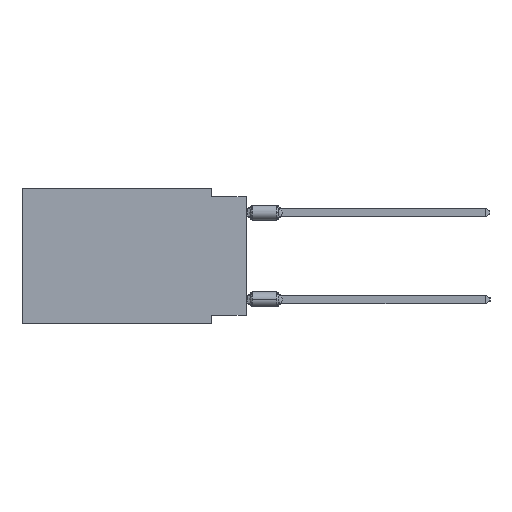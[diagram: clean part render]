
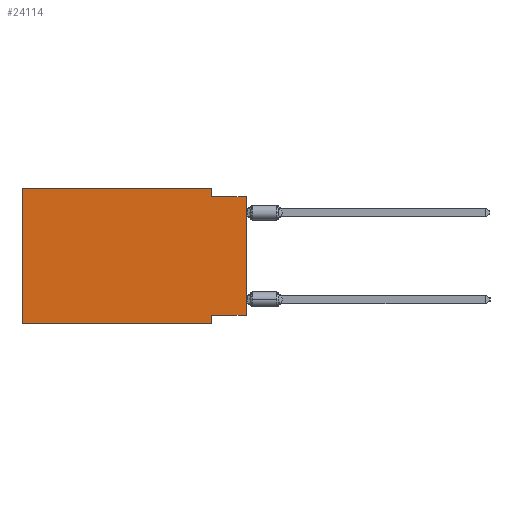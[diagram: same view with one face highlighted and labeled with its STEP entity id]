
A CAD part, left-side view. The second image highlights one B-rep face of the part: STEP entity #24114.
In plain terms, the highlighted planar face has unit normal (-1, 0, 0).
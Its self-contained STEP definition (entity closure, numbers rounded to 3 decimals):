
#54 = ORIENTED_EDGE ( 'NONE', *, *, #23808, .F. ) ;
#677 = VECTOR ( 'NONE', #4953, 1000. ) ;
#1441 = VERTEX_POINT ( 'NONE', #38375 ) ;
#1589 = LINE ( 'NONE', #32729, #54582 ) ;
#2730 = VERTEX_POINT ( 'NONE', #16091 ) ;
#4953 = DIRECTION ( 'NONE',  ( 0., 0., -1. ) ) ;
#5480 = DIRECTION ( 'NONE',  ( 0., -1., 0. ) ) ;
#6101 = ORIENTED_EDGE ( 'NONE', *, *, #49545, .F. ) ;
#6258 = EDGE_LOOP ( 'NONE', ( #31792, #54, #37159, #52309, #41253, #50559, #6101, #54483 ) ) ;
#8408 = CARTESIAN_POINT ( 'NONE',  ( 0., 0., -0.635 ) ) ;
#11209 = LINE ( 'NONE', #42965, #44977 ) ;
#12343 = VECTOR ( 'NONE', #34925, 1000. ) ;
#15864 = DIRECTION ( 'NONE',  ( 1., 0., 0. ) ) ;
#15942 = VECTOR ( 'NONE', #33941, 1000. ) ;
#16091 = CARTESIAN_POINT ( 'NONE',  ( 0., 2.54, 0. ) ) ;
#16144 = FACE_OUTER_BOUND ( 'NONE', #6258, .T. ) ;
#16253 = CARTESIAN_POINT ( 'NONE',  ( 0., 0., -0.635 ) ) ;
#19783 = CARTESIAN_POINT ( 'NONE',  ( 0., 0., -9.271 ) ) ;
#20161 = CARTESIAN_POINT ( 'NONE',  ( 0., 0., -9.271 ) ) ;
#20338 = LINE ( 'NONE', #52939, #46382 ) ;
#22613 = VECTOR ( 'NONE', #27285, 1000. ) ;
#23752 = VERTEX_POINT ( 'NONE', #25787 ) ;
#23808 = EDGE_CURVE ( 'NONE', #23752, #26547, #26990, .T. ) ;
#24114 = ADVANCED_FACE ( 'NONE', ( #16144 ), #25144, .F. ) ;
#24115 = CARTESIAN_POINT ( 'NONE',  ( 0., 16.383, -9.906 ) ) ;
#25144 = PLANE ( 'NONE',  #25330 ) ;
#25330 = AXIS2_PLACEMENT_3D ( 'NONE', #47614, #15864, #38909 ) ;
#25787 = CARTESIAN_POINT ( 'NONE',  ( 0., 2.54, -0.635 ) ) ;
#26547 = VERTEX_POINT ( 'NONE', #16253 ) ;
#26990 = LINE ( 'NONE', #8408, #22613 ) ;
#27131 = LINE ( 'NONE', #54372, #677 ) ;
#27285 = DIRECTION ( 'NONE',  ( 0., -1., 0. ) ) ;
#29143 = EDGE_CURVE ( 'NONE', #39453, #26547, #58256, .T. ) ;
#29194 = EDGE_CURVE ( 'NONE', #2730, #23752, #39709, .T. ) ;
#29446 = VERTEX_POINT ( 'NONE', #24115 ) ;
#31662 = VERTEX_POINT ( 'NONE', #49629 ) ;
#31792 = ORIENTED_EDGE ( 'NONE', *, *, #29143, .T. ) ;
#32729 = CARTESIAN_POINT ( 'NONE',  ( 0., 16.383, -9.906 ) ) ;
#33104 = DIRECTION ( 'NONE',  ( 0., -1., 0. ) ) ;
#33941 = DIRECTION ( 'NONE',  ( 0., 1., 0. ) ) ;
#34925 = DIRECTION ( 'NONE',  ( 0., 0., 1. ) ) ;
#36777 = EDGE_CURVE ( 'NONE', #31662, #2730, #11209, .T. ) ;
#37159 = ORIENTED_EDGE ( 'NONE', *, *, #29194, .F. ) ;
#37200 = VECTOR ( 'NONE', #57974, 1000. ) ;
#37273 = EDGE_CURVE ( 'NONE', #29446, #57665, #1589, .T. ) ;
#38375 = CARTESIAN_POINT ( 'NONE',  ( 0., 2.54, -9.271 ) ) ;
#38909 = DIRECTION ( 'NONE',  ( 0., 0., -1. ) ) ;
#39453 = VERTEX_POINT ( 'NONE', #19783 ) ;
#39709 = LINE ( 'NONE', #48101, #37200 ) ;
#41253 = ORIENTED_EDGE ( 'NONE', *, *, #45602, .F. ) ;
#42965 = CARTESIAN_POINT ( 'NONE',  ( 0., 16.383, 0. ) ) ;
#44259 = DIRECTION ( 'NONE',  ( 0., 0., 1. ) ) ;
#44977 = VECTOR ( 'NONE', #33104, 1000. ) ;
#45602 = EDGE_CURVE ( 'NONE', #29446, #31662, #20338, .T. ) ;
#46382 = VECTOR ( 'NONE', #44259, 1000. ) ;
#47614 = CARTESIAN_POINT ( 'NONE',  ( 0., 16.383, 0. ) ) ;
#48101 = CARTESIAN_POINT ( 'NONE',  ( 0., 2.54, 0. ) ) ;
#49371 = EDGE_CURVE ( 'NONE', #39453, #1441, #50997, .T. ) ;
#49545 = EDGE_CURVE ( 'NONE', #1441, #57665, #27131, .T. ) ;
#49629 = CARTESIAN_POINT ( 'NONE',  ( 0., 16.383, 0. ) ) ;
#50559 = ORIENTED_EDGE ( 'NONE', *, *, #37273, .T. ) ;
#50997 = LINE ( 'NONE', #20161, #15942 ) ;
#52309 = ORIENTED_EDGE ( 'NONE', *, *, #36777, .F. ) ;
#52442 = CARTESIAN_POINT ( 'NONE',  ( 0., 2.54, -9.906 ) ) ;
#52939 = CARTESIAN_POINT ( 'NONE',  ( 0., 16.383, 0. ) ) ;
#54372 = CARTESIAN_POINT ( 'NONE',  ( 0., 2.54, -9.906 ) ) ;
#54483 = ORIENTED_EDGE ( 'NONE', *, *, #49371, .F. ) ;
#54582 = VECTOR ( 'NONE', #5480, 1000. ) ;
#57089 = CARTESIAN_POINT ( 'NONE',  ( 0., 0., 0. ) ) ;
#57665 = VERTEX_POINT ( 'NONE', #52442 ) ;
#57974 = DIRECTION ( 'NONE',  ( 0., 0., -1. ) ) ;
#58256 = LINE ( 'NONE', #57089, #12343 ) ;
